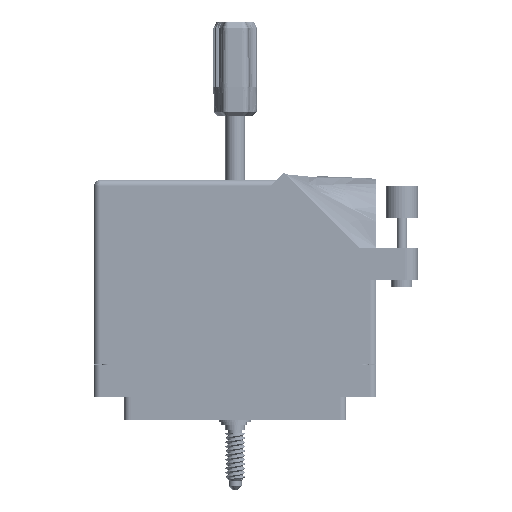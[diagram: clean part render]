
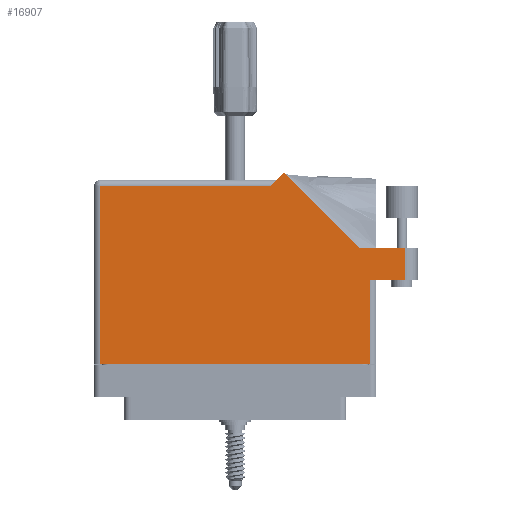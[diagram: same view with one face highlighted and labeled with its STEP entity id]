
A CAD part, front view. The second image highlights one B-rep face of the part: STEP entity #16907.
In plain terms, the highlighted face is planar.
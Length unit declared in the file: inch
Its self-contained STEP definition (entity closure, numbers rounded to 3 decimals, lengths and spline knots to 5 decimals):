
#718 = CARTESIAN_POINT ( 'NONE',  ( 0.46971, 1.74571, 0.617 ) ) ;
#3530 = VERTEX_POINT ( 'NONE', #18985 ) ;
#4998 = DIRECTION ( 'NONE',  ( 1., 0., 0. ) ) ;
#6895 = CARTESIAN_POINT ( 'NONE',  ( -1.359, -0.1, 0.617 ) ) ;
#7229 = VERTEX_POINT ( 'NONE', #718 ) ;
#8196 = ORIENTED_EDGE ( 'NONE', *, *, #85067, .T. ) ;
#8742 = ORIENTED_EDGE ( 'NONE', *, *, #56046, .T. ) ;
#12071 = CARTESIAN_POINT ( 'NONE',  ( -1.359, 1.613, 0.617 ) ) ;
#13720 = DIRECTION ( 'NONE',  ( -0.707, 0.707, 0. ) ) ;
#14030 = VECTOR ( 'NONE', #77378, 39.37008 ) ;
#15276 = VECTOR ( 'NONE', #35129, 39.37008 ) ;
#15430 = ORIENTED_EDGE ( 'NONE', *, *, #56898, .T. ) ;
#16266 = VERTEX_POINT ( 'NONE', #49487 ) ;
#16747 = CARTESIAN_POINT ( 'NONE',  ( -1.359, 1.675, 0.617 ) ) ;
#16907 = ADVANCED_FACE ( 'NONE', ( #18271 ), #43539, .F. ) ;
#17048 = EDGE_CURVE ( 'NONE', #69811, #62679, #70754, .T. ) ;
#18271 = FACE_OUTER_BOUND ( 'NONE', #69151, .T. ) ;
#18630 = LINE ( 'NONE', #25970, #35431 ) ;
#18985 = CARTESIAN_POINT ( 'NONE',  ( -1.297, -0.1, 0.617 ) ) ;
#22643 = CARTESIAN_POINT ( 'NONE',  ( 1.19342, 1.022, 0.617 ) ) ;
#23106 = CARTESIAN_POINT ( 'NONE',  ( 0.337, 1.613, 0.617 ) ) ;
#25376 = DIRECTION ( 'NONE',  ( 0., 1., 0. ) ) ;
#25970 = CARTESIAN_POINT ( 'NONE',  ( 1.634, 1.022, 0.617 ) ) ;
#27035 = ORIENTED_EDGE ( 'NONE', *, *, #59917, .T. ) ;
#28333 = EDGE_CURVE ( 'NONE', #62679, #3530, #69687, .T. ) ;
#29637 = DIRECTION ( 'NONE',  ( -1., 0., 0. ) ) ;
#30226 = DIRECTION ( 'NONE',  ( 0., 0., -1. ) ) ;
#30955 = VERTEX_POINT ( 'NONE', #85518 ) ;
#32631 = ORIENTED_EDGE ( 'NONE', *, *, #33370, .T. ) ;
#33370 = EDGE_CURVE ( 'NONE', #30955, #82410, #86654, .T. ) ;
#35129 = DIRECTION ( 'NONE',  ( -1., 0., 0. ) ) ;
#35431 = VECTOR ( 'NONE', #25376, 39.37008 ) ;
#41231 = DIRECTION ( 'NONE',  ( 1., 0., 0. ) ) ;
#41642 = CARTESIAN_POINT ( 'NONE',  ( -1.297, 1.613, 0.617 ) ) ;
#42717 = EDGE_CURVE ( 'NONE', #7229, #69811, #51036, .T. ) ;
#43312 = LINE ( 'NONE', #53938, #50595 ) ;
#43539 = PLANE ( 'NONE',  #43826 ) ;
#43826 = AXIS2_PLACEMENT_3D ( 'NONE', #16747, #30226, #29637 ) ;
#44733 = ORIENTED_EDGE ( 'NONE', *, *, #17048, .T. ) ;
#46321 = DIRECTION ( 'NONE',  ( -0.707, -0.707, 0. ) ) ;
#48307 = ORIENTED_EDGE ( 'NONE', *, *, #51037, .T. ) ;
#48951 = VECTOR ( 'NONE', #41231, 39.37008 ) ;
#49487 = CARTESIAN_POINT ( 'NONE',  ( 1.297, -0.1, 0.617 ) ) ;
#50595 = VECTOR ( 'NONE', #13720, 39.37008 ) ;
#51036 = LINE ( 'NONE', #79735, #72006 ) ;
#51037 = EDGE_CURVE ( 'NONE', #51800, #30955, #18630, .T. ) ;
#51622 = CARTESIAN_POINT ( 'NONE',  ( 1.359, 0.715, 0.617 ) ) ;
#51689 = DIRECTION ( 'NONE',  ( -1., 0., 0. ) ) ;
#51800 = VERTEX_POINT ( 'NONE', #52727 ) ;
#51856 = LINE ( 'NONE', #65145, #67588 ) ;
#52727 = CARTESIAN_POINT ( 'NONE',  ( 1.634, 0.715, 0.617 ) ) ;
#52975 = VECTOR ( 'NONE', #51689, 39.37008 ) ;
#53938 = CARTESIAN_POINT ( 'NONE',  ( 1.19342, 1.022, 0.617 ) ) ;
#55975 = LINE ( 'NONE', #51622, #67481 ) ;
#56046 = EDGE_CURVE ( 'NONE', #64084, #51800, #55975, .T. ) ;
#56898 = EDGE_CURVE ( 'NONE', #82410, #7229, #43312, .T. ) ;
#59917 = EDGE_CURVE ( 'NONE', #3530, #16266, #73094, .T. ) ;
#61614 = CARTESIAN_POINT ( 'NONE',  ( 1.759, 1.022, 0.617 ) ) ;
#62679 = VERTEX_POINT ( 'NONE', #41642 ) ;
#64084 = VERTEX_POINT ( 'NONE', #77744 ) ;
#65145 = CARTESIAN_POINT ( 'NONE',  ( 1.297, 0.715, 0.617 ) ) ;
#67394 = ORIENTED_EDGE ( 'NONE', *, *, #42717, .T. ) ;
#67481 = VECTOR ( 'NONE', #4998, 39.37008 ) ;
#67588 = VECTOR ( 'NONE', #78594, 39.37008 ) ;
#69151 = EDGE_LOOP ( 'NONE', ( #8742, #48307, #32631, #15430, #67394, #44733, #82548, #27035, #8196 ) ) ;
#69687 = LINE ( 'NONE', #83540, #14030 ) ;
#69811 = VERTEX_POINT ( 'NONE', #23106 ) ;
#70754 = LINE ( 'NONE', #12071, #52975 ) ;
#72006 = VECTOR ( 'NONE', #46321, 39.37008 ) ;
#73094 = LINE ( 'NONE', #6895, #48951 ) ;
#77378 = DIRECTION ( 'NONE',  ( 0., -1., 0. ) ) ;
#77744 = CARTESIAN_POINT ( 'NONE',  ( 1.297, 0.715, 0.617 ) ) ;
#78594 = DIRECTION ( 'NONE',  ( 0., 1., 0. ) ) ;
#79735 = CARTESIAN_POINT ( 'NONE',  ( 0.399, 1.675, 0.617 ) ) ;
#82410 = VERTEX_POINT ( 'NONE', #22643 ) ;
#82548 = ORIENTED_EDGE ( 'NONE', *, *, #28333, .T. ) ;
#83540 = CARTESIAN_POINT ( 'NONE',  ( -1.297, -0.1, 0.617 ) ) ;
#85067 = EDGE_CURVE ( 'NONE', #16266, #64084, #51856, .T. ) ;
#85518 = CARTESIAN_POINT ( 'NONE',  ( 1.634, 1.022, 0.617 ) ) ;
#86654 = LINE ( 'NONE', #61614, #15276 ) ;
